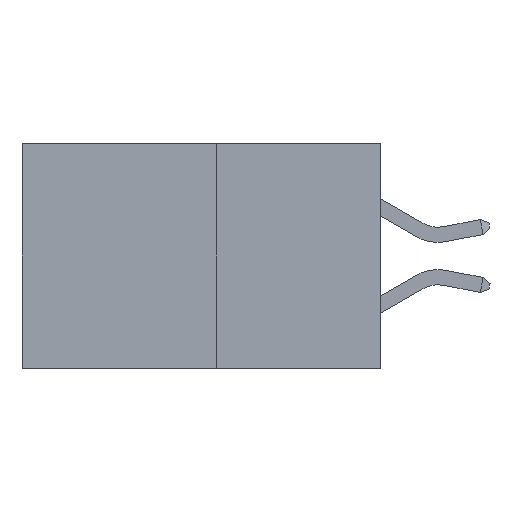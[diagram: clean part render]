
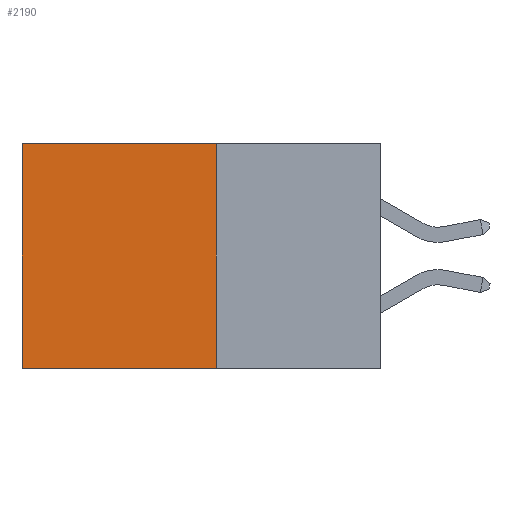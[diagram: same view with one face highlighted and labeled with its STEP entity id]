
A CAD part, left-side view. The second image highlights one B-rep face of the part: STEP entity #2190.
In plain terms, the highlighted planar face has unit normal (-1, 0, 0).
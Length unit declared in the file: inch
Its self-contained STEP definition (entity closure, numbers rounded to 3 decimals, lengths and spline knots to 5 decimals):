
#34 = EDGE_CURVE ( 'NONE', #4675, #3671, #7690, .T. ) ;
#284 = DIRECTION ( 'NONE',  ( 0., 0., -1. ) ) ;
#294 = ORIENTED_EDGE ( 'NONE', *, *, #5160, .T. ) ;
#356 = DIRECTION ( 'NONE',  ( 0., 0., -1. ) ) ;
#618 = EDGE_CURVE ( 'NONE', #7239, #4675, #5823, .T. ) ;
#717 = DIRECTION ( 'NONE',  ( 0., 1., 0. ) ) ;
#940 = ORIENTED_EDGE ( 'NONE', *, *, #8876, .T. ) ;
#1189 = CARTESIAN_POINT ( 'NONE',  ( 0.277, 0.27, -0.37 ) ) ;
#2190 = ADVANCED_FACE ( 'NONE', ( #6975 ), #3978, .F. ) ;
#2827 = VECTOR ( 'NONE', #717, 39.37008 ) ;
#2890 = DIRECTION ( 'NONE',  ( 1., 0., 0. ) ) ;
#3086 = ORIENTED_EDGE ( 'NONE', *, *, #618, .F. ) ;
#3148 = VECTOR ( 'NONE', #4566, 39.37008 ) ;
#3304 = CARTESIAN_POINT ( 'NONE',  ( 0.277, 0.59, 0. ) ) ;
#3410 = DIRECTION ( 'NONE',  ( 0., 1., 0. ) ) ;
#3415 = CARTESIAN_POINT ( 'NONE',  ( 0.277, 0.27, -0.37 ) ) ;
#3671 = VERTEX_POINT ( 'NONE', #7873 ) ;
#3841 = CARTESIAN_POINT ( 'NONE',  ( 0.277, 0.59, -0.37 ) ) ;
#3978 = PLANE ( 'NONE',  #4187 ) ;
#4187 = AXIS2_PLACEMENT_3D ( 'NONE', #1189, #2890, #356 ) ;
#4566 = DIRECTION ( 'NONE',  ( 0., 0., -1. ) ) ;
#4675 = VERTEX_POINT ( 'NONE', #3415 ) ;
#5160 = EDGE_CURVE ( 'NONE', #5654, #3671, #5572, .T. ) ;
#5572 = LINE ( 'NONE', #3841, #3148 ) ;
#5654 = VERTEX_POINT ( 'NONE', #3304 ) ;
#5823 = LINE ( 'NONE', #8956, #9631 ) ;
#6975 = FACE_OUTER_BOUND ( 'NONE', #8111, .T. ) ;
#7239 = VERTEX_POINT ( 'NONE', #10543 ) ;
#7348 = LINE ( 'NONE', #9647, #2827 ) ;
#7444 = VECTOR ( 'NONE', #3410, 39.37008 ) ;
#7690 = LINE ( 'NONE', #7717, #7444 ) ;
#7717 = CARTESIAN_POINT ( 'NONE',  ( 0.277, 0.27, -0.37 ) ) ;
#7873 = CARTESIAN_POINT ( 'NONE',  ( 0.277, 0.59, -0.37 ) ) ;
#8111 = EDGE_LOOP ( 'NONE', ( #294, #9140, #3086, #940 ) ) ;
#8876 = EDGE_CURVE ( 'NONE', #7239, #5654, #7348, .T. ) ;
#8956 = CARTESIAN_POINT ( 'NONE',  ( 0.277, 0.27, -0.37 ) ) ;
#9140 = ORIENTED_EDGE ( 'NONE', *, *, #34, .F. ) ;
#9631 = VECTOR ( 'NONE', #284, 39.37008 ) ;
#9647 = CARTESIAN_POINT ( 'NONE',  ( 0.277, 0.27, 0. ) ) ;
#10543 = CARTESIAN_POINT ( 'NONE',  ( 0.277, 0.27, 0. ) ) ;
